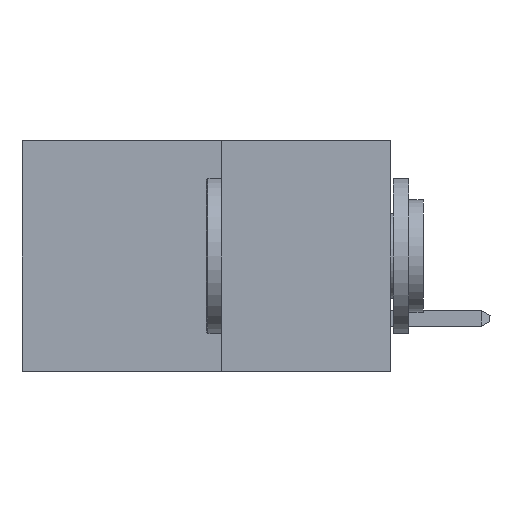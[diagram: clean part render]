
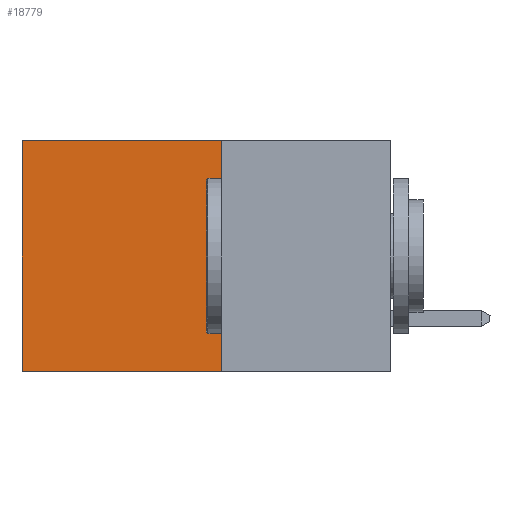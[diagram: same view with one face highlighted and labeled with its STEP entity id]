
A CAD part, left-side view. The second image highlights one B-rep face of the part: STEP entity #18779.
In plain terms, the highlighted planar face has unit normal (-1, 0, 0).
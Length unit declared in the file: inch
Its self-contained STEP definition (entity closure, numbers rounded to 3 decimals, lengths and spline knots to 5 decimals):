
#163 = FACE_OUTER_BOUND ( 'NONE', #8308, .T. ) ;
#577 = LINE ( 'NONE', #13763, #11418 ) ;
#924 = PLANE ( 'NONE',  #15179 ) ;
#1308 = VECTOR ( 'NONE', #8138, 39.37008 ) ;
#1761 = ORIENTED_EDGE ( 'NONE', *, *, #5449, .F. ) ;
#1943 = VERTEX_POINT ( 'NONE', #3411 ) ;
#2472 = LINE ( 'NONE', #17098, #13633 ) ;
#2506 = CARTESIAN_POINT ( 'NONE',  ( 0.277, 0.27, -0.37 ) ) ;
#3081 = LINE ( 'NONE', #7881, #6730 ) ;
#3411 = CARTESIAN_POINT ( 'NONE',  ( 0.277, 0.27, -0.37 ) ) ;
#3771 = DIRECTION ( 'NONE',  ( 0., 0., -1. ) ) ;
#4879 = EDGE_CURVE ( 'NONE', #1943, #5375, #3081, .T. ) ;
#4963 = ORIENTED_EDGE ( 'NONE', *, *, #4879, .F. ) ;
#5375 = VERTEX_POINT ( 'NONE', #17934 ) ;
#5449 = EDGE_CURVE ( 'NONE', #13361, #1943, #577, .T. ) ;
#5571 = EDGE_CURVE ( 'NONE', #13361, #10891, #13004, .T. ) ;
#5672 = DIRECTION ( 'NONE',  ( 0., 0., -1. ) ) ;
#6730 = VECTOR ( 'NONE', #8377, 39.37008 ) ;
#7881 = CARTESIAN_POINT ( 'NONE',  ( 0.277, 0.27, -0.37 ) ) ;
#8138 = DIRECTION ( 'NONE',  ( 0., 1., 0. ) ) ;
#8308 = EDGE_LOOP ( 'NONE', ( #14566, #4963, #1761, #14361 ) ) ;
#8377 = DIRECTION ( 'NONE',  ( 0., 1., 0. ) ) ;
#10891 = VERTEX_POINT ( 'NONE', #12156 ) ;
#11418 = VECTOR ( 'NONE', #15203, 39.37008 ) ;
#12156 = CARTESIAN_POINT ( 'NONE',  ( 0.277, 0.59, 0. ) ) ;
#13004 = LINE ( 'NONE', #16872, #1308 ) ;
#13361 = VERTEX_POINT ( 'NONE', #17921 ) ;
#13633 = VECTOR ( 'NONE', #3771, 39.37008 ) ;
#13763 = CARTESIAN_POINT ( 'NONE',  ( 0.277, 0.27, -0.37 ) ) ;
#14338 = EDGE_CURVE ( 'NONE', #10891, #5375, #2472, .T. ) ;
#14361 = ORIENTED_EDGE ( 'NONE', *, *, #5571, .T. ) ;
#14566 = ORIENTED_EDGE ( 'NONE', *, *, #14338, .T. ) ;
#14605 = DIRECTION ( 'NONE',  ( 1., 0., 0. ) ) ;
#15179 = AXIS2_PLACEMENT_3D ( 'NONE', #2506, #14605, #5672 ) ;
#15203 = DIRECTION ( 'NONE',  ( 0., 0., -1. ) ) ;
#16872 = CARTESIAN_POINT ( 'NONE',  ( 0.277, 0.27, 0. ) ) ;
#17098 = CARTESIAN_POINT ( 'NONE',  ( 0.277, 0.59, -0.37 ) ) ;
#17921 = CARTESIAN_POINT ( 'NONE',  ( 0.277, 0.27, 0. ) ) ;
#17934 = CARTESIAN_POINT ( 'NONE',  ( 0.277, 0.59, -0.37 ) ) ;
#18779 = ADVANCED_FACE ( 'NONE', ( #163 ), #924, .F. ) ;
